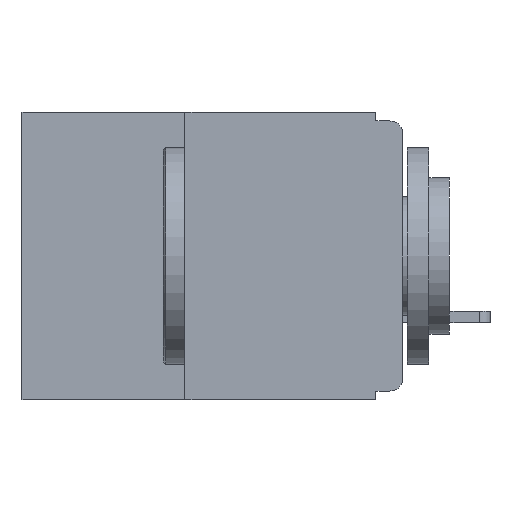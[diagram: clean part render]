
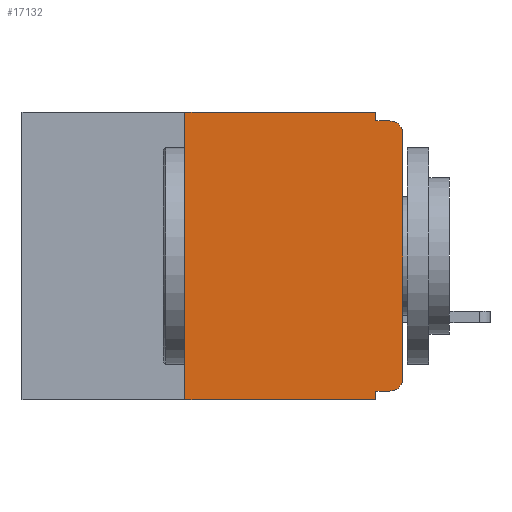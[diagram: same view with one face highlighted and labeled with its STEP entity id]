
A CAD part, left-side view. The second image highlights one B-rep face of the part: STEP entity #17132.
In plain terms, the highlighted planar face has unit normal (-1, 0, 0).
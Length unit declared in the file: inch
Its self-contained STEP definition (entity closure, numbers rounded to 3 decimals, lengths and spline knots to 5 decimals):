
#82 = ORIENTED_EDGE ( 'NONE', *, *, #10187, .F. ) ;
#251 = CARTESIAN_POINT ( 'NONE',  ( 0., 0.25, 0. ) ) ;
#419 = DIRECTION ( 'NONE',  ( 0., 0., -1. ) ) ;
#1110 = CARTESIAN_POINT ( 'NONE',  ( 0., 0.031, 0. ) ) ;
#1172 = ORIENTED_EDGE ( 'NONE', *, *, #9517, .T. ) ;
#1500 = DIRECTION ( 'NONE',  ( -1., 0., 0. ) ) ;
#1851 = VECTOR ( 'NONE', #419, 39.37008 ) ;
#1968 = EDGE_CURVE ( 'NONE', #5391, #22697, #12075, .T. ) ;
#2004 = DIRECTION ( 'NONE',  ( 1., 0., 0. ) ) ;
#3708 = LINE ( 'NONE', #6440, #8384 ) ;
#3929 = CARTESIAN_POINT ( 'NONE',  ( 0., 0., 0. ) ) ;
#4011 = CIRCLE ( 'NONE', #8342, 0.015 ) ;
#4031 = ORIENTED_EDGE ( 'NONE', *, *, #16640, .F. ) ;
#4301 = DIRECTION ( 'NONE',  ( 0., 0., 1. ) ) ;
#4707 = CARTESIAN_POINT ( 'NONE',  ( 0., 0., -0.025 ) ) ;
#5391 = VERTEX_POINT ( 'NONE', #19648 ) ;
#6440 = CARTESIAN_POINT ( 'NONE',  ( 0., 0.25, -0.33 ) ) ;
#6549 = DIRECTION ( 'NONE',  ( 0., 0., 1. ) ) ;
#6712 = EDGE_CURVE ( 'NONE', #27405, #15760, #12254, .T. ) ;
#7026 = LINE ( 'NONE', #17269, #24505 ) ;
#7083 = DIRECTION ( 'NONE',  ( 0., 0., -1. ) ) ;
#7445 = EDGE_CURVE ( 'NONE', #25035, #9972, #27876, .T. ) ;
#7994 = LINE ( 'NONE', #14081, #1851 ) ;
#8175 = VERTEX_POINT ( 'NONE', #19885 ) ;
#8342 = AXIS2_PLACEMENT_3D ( 'NONE', #15253, #1500, #17542 ) ;
#8384 = VECTOR ( 'NONE', #6549, 39.37008 ) ;
#9517 = EDGE_CURVE ( 'NONE', #9622, #11172, #9605, .T. ) ;
#9605 = LINE ( 'NONE', #19932, #14239 ) ;
#9622 = VERTEX_POINT ( 'NONE', #20327 ) ;
#9767 = ORIENTED_EDGE ( 'NONE', *, *, #29511, .T. ) ;
#9972 = VERTEX_POINT ( 'NONE', #1110 ) ;
#10187 = EDGE_CURVE ( 'NONE', #9622, #25035, #3708, .T. ) ;
#10680 = CARTESIAN_POINT ( 'NONE',  ( 0., 0.015, -0.305 ) ) ;
#10907 = DIRECTION ( 'NONE',  ( 0., -1., 0. ) ) ;
#11172 = VERTEX_POINT ( 'NONE', #12808 ) ;
#11582 = EDGE_CURVE ( 'NONE', #15760, #11172, #7994, .T. ) ;
#11933 = CARTESIAN_POINT ( 'NONE',  ( 0., 0., -0.32 ) ) ;
#12075 = LINE ( 'NONE', #3929, #29538 ) ;
#12254 = LINE ( 'NONE', #11933, #23640 ) ;
#12808 = CARTESIAN_POINT ( 'NONE',  ( 0., 0.031, -0.33 ) ) ;
#12953 = CARTESIAN_POINT ( 'NONE',  ( 0., 0.031, -0.32 ) ) ;
#12988 = DIRECTION ( 'NONE',  ( 0., 0., -1. ) ) ;
#12996 = VERTEX_POINT ( 'NONE', #28805 ) ;
#13770 = EDGE_LOOP ( 'NONE', ( #22573, #9767, #15489, #4031, #25493, #82, #1172, #21589, #17684, #20334 ) ) ;
#13888 = CARTESIAN_POINT ( 'NONE',  ( 0., 0.031, 0. ) ) ;
#14081 = CARTESIAN_POINT ( 'NONE',  ( 0., 0.031, -0.33 ) ) ;
#14210 = DIRECTION ( 'NONE',  ( 0., 1., 0. ) ) ;
#14239 = VECTOR ( 'NONE', #10907, 39.37008 ) ;
#15253 = CARTESIAN_POINT ( 'NONE',  ( 0., 0.015, -0.025 ) ) ;
#15489 = ORIENTED_EDGE ( 'NONE', *, *, #22997, .F. ) ;
#15617 = CARTESIAN_POINT ( 'NONE',  ( 0., 0.015, -0.32 ) ) ;
#15760 = VERTEX_POINT ( 'NONE', #12953 ) ;
#16640 = EDGE_CURVE ( 'NONE', #9972, #12996, #25807, .T. ) ;
#17132 = ADVANCED_FACE ( 'NONE', ( #22191 ), #29400, .F. ) ;
#17269 = CARTESIAN_POINT ( 'NONE',  ( 0., 0., -0.01 ) ) ;
#17542 = DIRECTION ( 'NONE',  ( 0., 0., -1. ) ) ;
#17684 = ORIENTED_EDGE ( 'NONE', *, *, #6712, .F. ) ;
#18033 = DIRECTION ( 'NONE',  ( 0., 0., -1. ) ) ;
#18601 = AXIS2_PLACEMENT_3D ( 'NONE', #10680, #26633, #12988 ) ;
#19551 = DIRECTION ( 'NONE',  ( 0., -1., 0. ) ) ;
#19648 = CARTESIAN_POINT ( 'NONE',  ( 0., 0., -0.305 ) ) ;
#19885 = CARTESIAN_POINT ( 'NONE',  ( 0., 0.015, -0.01 ) ) ;
#19932 = CARTESIAN_POINT ( 'NONE',  ( 0., 0.437, -0.33 ) ) ;
#20327 = CARTESIAN_POINT ( 'NONE',  ( 0., 0.25, -0.33 ) ) ;
#20334 = ORIENTED_EDGE ( 'NONE', *, *, #26612, .T. ) ;
#21589 = ORIENTED_EDGE ( 'NONE', *, *, #11582, .F. ) ;
#21809 = VECTOR ( 'NONE', #26346, 39.37008 ) ;
#22191 = FACE_OUTER_BOUND ( 'NONE', #13770, .T. ) ;
#22510 = CARTESIAN_POINT ( 'NONE',  ( 0., 0.437, 0. ) ) ;
#22573 = ORIENTED_EDGE ( 'NONE', *, *, #1968, .T. ) ;
#22697 = VERTEX_POINT ( 'NONE', #4707 ) ;
#22997 = EDGE_CURVE ( 'NONE', #12996, #8175, #7026, .T. ) ;
#23640 = VECTOR ( 'NONE', #14210, 39.37008 ) ;
#24040 = CARTESIAN_POINT ( 'NONE',  ( 0., 0.437, 0. ) ) ;
#24505 = VECTOR ( 'NONE', #19551, 39.37008 ) ;
#25035 = VERTEX_POINT ( 'NONE', #251 ) ;
#25093 = VECTOR ( 'NONE', #7083, 39.37008 ) ;
#25348 = CIRCLE ( 'NONE', #18601, 0.015 ) ;
#25493 = ORIENTED_EDGE ( 'NONE', *, *, #7445, .F. ) ;
#25807 = LINE ( 'NONE', #13888, #25093 ) ;
#26346 = DIRECTION ( 'NONE',  ( 0., -1., 0. ) ) ;
#26612 = EDGE_CURVE ( 'NONE', #27405, #5391, #25348, .T. ) ;
#26633 = DIRECTION ( 'NONE',  ( -1., 0., 0. ) ) ;
#27405 = VERTEX_POINT ( 'NONE', #15617 ) ;
#27876 = LINE ( 'NONE', #24040, #21809 ) ;
#28805 = CARTESIAN_POINT ( 'NONE',  ( 0., 0.031, -0.01 ) ) ;
#28998 = AXIS2_PLACEMENT_3D ( 'NONE', #22510, #2004, #18033 ) ;
#29400 = PLANE ( 'NONE',  #28998 ) ;
#29511 = EDGE_CURVE ( 'NONE', #22697, #8175, #4011, .T. ) ;
#29538 = VECTOR ( 'NONE', #4301, 39.37008 ) ;
